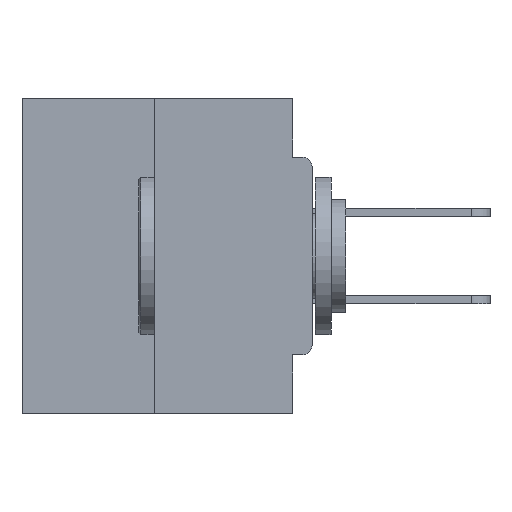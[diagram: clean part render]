
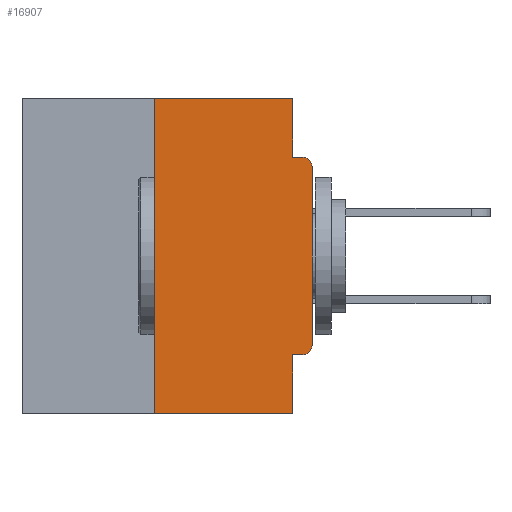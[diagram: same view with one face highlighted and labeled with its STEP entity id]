
A CAD part, left-side view. The second image highlights one B-rep face of the part: STEP entity #16907.
In plain terms, the highlighted planar face has unit normal (-1, 0, 0).
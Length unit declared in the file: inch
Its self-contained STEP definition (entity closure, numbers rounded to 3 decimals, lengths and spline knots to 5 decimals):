
#843 = VERTEX_POINT ( 'NONE', #30806 ) ;
#1064 = VECTOR ( 'NONE', #1233, 39.37008 ) ;
#1214 = CARTESIAN_POINT ( 'NONE',  ( 0., 0.031, -0.4065 ) ) ;
#1233 = DIRECTION ( 'NONE',  ( 0., -1., 0. ) ) ;
#1342 = CARTESIAN_POINT ( 'NONE',  ( 0., 0.46, 0. ) ) ;
#1384 = VECTOR ( 'NONE', #7371, 39.37008 ) ;
#1549 = LINE ( 'NONE', #4855, #15977 ) ;
#1819 = CIRCLE ( 'NONE', #10115, 0.015 ) ;
#3059 = LINE ( 'NONE', #9154, #1064 ) ;
#3213 = PLANE ( 'NONE',  #3936 ) ;
#3234 = DIRECTION ( 'NONE',  ( 0., 0., 1. ) ) ;
#3445 = CARTESIAN_POINT ( 'NONE',  ( 0., 0.015, -0.4065 ) ) ;
#3781 = VERTEX_POINT ( 'NONE', #9126 ) ;
#3936 = AXIS2_PLACEMENT_3D ( 'NONE', #28817, #13496, #26008 ) ;
#4855 = CARTESIAN_POINT ( 'NONE',  ( 0., 0., -0.4065 ) ) ;
#5083 = EDGE_CURVE ( 'NONE', #20400, #7942, #3059, .T. ) ;
#5107 = VERTEX_POINT ( 'NONE', #19405 ) ;
#5166 = LINE ( 'NONE', #13624, #21999 ) ;
#5315 = ORIENTED_EDGE ( 'NONE', *, *, #28866, .F. ) ;
#5378 = ORIENTED_EDGE ( 'NONE', *, *, #5583, .T. ) ;
#5583 = EDGE_CURVE ( 'NONE', #14306, #30093, #1819, .T. ) ;
#5659 = ORIENTED_EDGE ( 'NONE', *, *, #5083, .T. ) ;
#6262 = EDGE_CURVE ( 'NONE', #843, #30746, #11402, .T. ) ;
#7371 = DIRECTION ( 'NONE',  ( 0., -1., 0. ) ) ;
#7591 = CARTESIAN_POINT ( 'NONE',  ( 0., 0., -0.3915 ) ) ;
#7601 = CARTESIAN_POINT ( 'NONE',  ( 0., 0., -0.0935 ) ) ;
#7783 = CARTESIAN_POINT ( 'NONE',  ( 0., 0.031, 0. ) ) ;
#7942 = VERTEX_POINT ( 'NONE', #17315 ) ;
#8307 = CARTESIAN_POINT ( 'NONE',  ( 0., 0.25, 0. ) ) ;
#9126 = CARTESIAN_POINT ( 'NONE',  ( 0., 0., -0.1085 ) ) ;
#9154 = CARTESIAN_POINT ( 'NONE',  ( 0., 0.46, -0.5 ) ) ;
#9651 = DIRECTION ( 'NONE',  ( 0., 1., 0. ) ) ;
#10115 = AXIS2_PLACEMENT_3D ( 'NONE', #24537, #19321, #27099 ) ;
#10201 = EDGE_CURVE ( 'NONE', #32137, #5107, #13362, .T. ) ;
#11402 = LINE ( 'NONE', #1342, #1384 ) ;
#11459 = LINE ( 'NONE', #15245, #14288 ) ;
#12873 = DIRECTION ( 'NONE',  ( 0., 0., -1. ) ) ;
#13362 = LINE ( 'NONE', #7601, #31367 ) ;
#13496 = DIRECTION ( 'NONE',  ( 1., 0., 0. ) ) ;
#13624 = CARTESIAN_POINT ( 'NONE',  ( 0., 0., 0. ) ) ;
#14108 = EDGE_LOOP ( 'NONE', ( #30977, #21363, #5659, #14487, #32538, #5378, #28352, #27526, #25509, #5315 ) ) ;
#14288 = VECTOR ( 'NONE', #12873, 39.37008 ) ;
#14306 = VERTEX_POINT ( 'NONE', #3445 ) ;
#14487 = ORIENTED_EDGE ( 'NONE', *, *, #25384, .F. ) ;
#15245 = CARTESIAN_POINT ( 'NONE',  ( 0., 0.031, -0.5 ) ) ;
#15346 = DIRECTION ( 'NONE',  ( 0., -1., 0. ) ) ;
#15977 = VECTOR ( 'NONE', #9651, 39.37008 ) ;
#16191 = EDGE_CURVE ( 'NONE', #20400, #843, #21373, .T. ) ;
#16860 = DIRECTION ( 'NONE',  ( 0., 0., -1. ) ) ;
#16907 = ADVANCED_FACE ( 'NONE', ( #20583 ), #3213, .F. ) ;
#17172 = VERTEX_POINT ( 'NONE', #1214 ) ;
#17272 = DIRECTION ( 'NONE',  ( 0., 0., -1. ) ) ;
#17315 = CARTESIAN_POINT ( 'NONE',  ( 0., 0.031, -0.5 ) ) ;
#19306 = EDGE_CURVE ( 'NONE', #14306, #17172, #1549, .T. ) ;
#19321 = DIRECTION ( 'NONE',  ( -1., 0., 0. ) ) ;
#19405 = CARTESIAN_POINT ( 'NONE',  ( 0., 0.015, -0.0935 ) ) ;
#19429 = EDGE_CURVE ( 'NONE', #30093, #3781, #5166, .T. ) ;
#20400 = VERTEX_POINT ( 'NONE', #28000 ) ;
#20583 = FACE_OUTER_BOUND ( 'NONE', #14108, .T. ) ;
#21363 = ORIENTED_EDGE ( 'NONE', *, *, #16191, .F. ) ;
#21373 = LINE ( 'NONE', #8307, #21775 ) ;
#21775 = VECTOR ( 'NONE', #31677, 39.37008 ) ;
#21999 = VECTOR ( 'NONE', #3234, 39.37008 ) ;
#24302 = CIRCLE ( 'NONE', #29257, 0.015 ) ;
#24537 = CARTESIAN_POINT ( 'NONE',  ( 0., 0.015, -0.3915 ) ) ;
#25172 = EDGE_CURVE ( 'NONE', #3781, #5107, #24302, .T. ) ;
#25384 = EDGE_CURVE ( 'NONE', #17172, #7942, #11459, .T. ) ;
#25509 = ORIENTED_EDGE ( 'NONE', *, *, #10201, .F. ) ;
#26008 = DIRECTION ( 'NONE',  ( 0., 0., -1. ) ) ;
#27099 = DIRECTION ( 'NONE',  ( 0., 0., -1. ) ) ;
#27304 = DIRECTION ( 'NONE',  ( -1., 0., 0. ) ) ;
#27526 = ORIENTED_EDGE ( 'NONE', *, *, #25172, .T. ) ;
#27939 = LINE ( 'NONE', #29801, #29988 ) ;
#28000 = CARTESIAN_POINT ( 'NONE',  ( 0., 0.25, -0.5 ) ) ;
#28352 = ORIENTED_EDGE ( 'NONE', *, *, #19429, .T. ) ;
#28817 = CARTESIAN_POINT ( 'NONE',  ( 0., 0.46, 0. ) ) ;
#28866 = EDGE_CURVE ( 'NONE', #30746, #32137, #27939, .T. ) ;
#29220 = CARTESIAN_POINT ( 'NONE',  ( 0., 0.015, -0.1085 ) ) ;
#29257 = AXIS2_PLACEMENT_3D ( 'NONE', #29220, #27304, #17272 ) ;
#29801 = CARTESIAN_POINT ( 'NONE',  ( 0., 0.031, 0. ) ) ;
#29988 = VECTOR ( 'NONE', #16860, 39.37008 ) ;
#30093 = VERTEX_POINT ( 'NONE', #7591 ) ;
#30746 = VERTEX_POINT ( 'NONE', #7783 ) ;
#30806 = CARTESIAN_POINT ( 'NONE',  ( 0., 0.25, 0. ) ) ;
#30977 = ORIENTED_EDGE ( 'NONE', *, *, #6262, .F. ) ;
#31367 = VECTOR ( 'NONE', #15346, 39.37008 ) ;
#31677 = DIRECTION ( 'NONE',  ( 0., 0., 1. ) ) ;
#31739 = CARTESIAN_POINT ( 'NONE',  ( 0., 0.031, -0.0935 ) ) ;
#32137 = VERTEX_POINT ( 'NONE', #31739 ) ;
#32538 = ORIENTED_EDGE ( 'NONE', *, *, #19306, .F. ) ;
